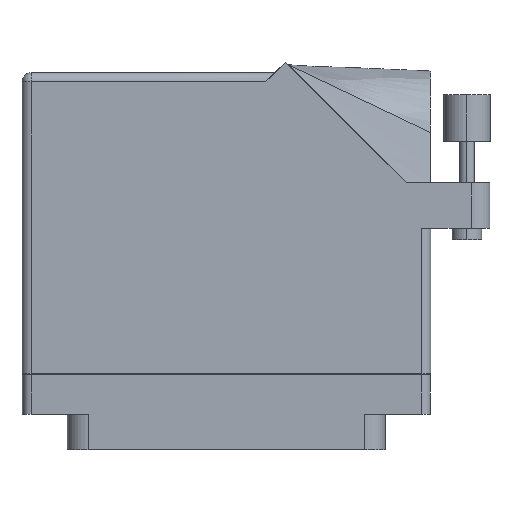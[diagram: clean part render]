
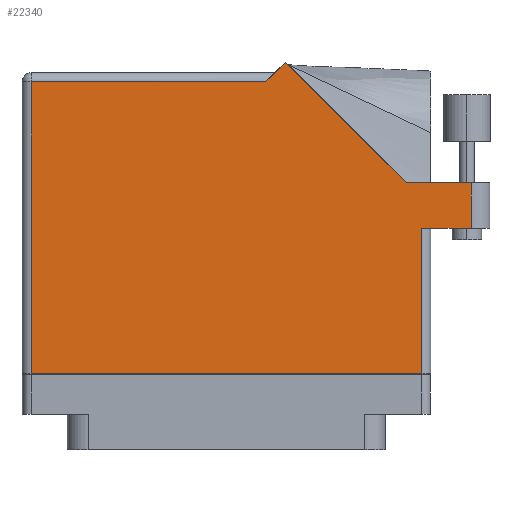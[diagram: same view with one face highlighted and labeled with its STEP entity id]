
A CAD part, front view. The second image highlights one B-rep face of the part: STEP entity #22340.
In plain terms, the highlighted face is planar.
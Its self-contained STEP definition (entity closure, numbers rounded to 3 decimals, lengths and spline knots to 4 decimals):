
#515 = CARTESIAN_POINT ( 'NONE',  ( 1.3155, 0.88, 0.765 ) ) ;
#1029 = CARTESIAN_POINT ( 'NONE',  ( 1.6525, 1.187, 0.765 ) ) ;
#1926 = DIRECTION ( 'NONE',  ( -1., 0., 0. ) ) ;
#1939 = VERTEX_POINT ( 'NONE', #44966 ) ;
#4307 = AXIS2_PLACEMENT_3D ( 'NONE', #61878, #61577, #21352 ) ;
#4882 = DIRECTION ( 'NONE',  ( -1., 0., 0. ) ) ;
#7314 = CARTESIAN_POINT ( 'NONE',  ( 1.6525, 0.88, 0.765 ) ) ;
#7640 = EDGE_CURVE ( 'NONE', #12763, #30041, #14751, .T. ) ;
#8707 = VERTEX_POINT ( 'NONE', #49635 ) ;
#8790 = VERTEX_POINT ( 'NONE', #7314 ) ;
#11628 = ORIENTED_EDGE ( 'NONE', *, *, #56207, .T. ) ;
#12763 = VERTEX_POINT ( 'NONE', #23673 ) ;
#14067 = PLANE ( 'NONE',  #4307 ) ;
#14723 = LINE ( 'NONE', #55177, #56525 ) ;
#14751 = LINE ( 'NONE', #14753, #34560 ) ;
#14753 = CARTESIAN_POINT ( 'NONE',  ( 1.7775, 1.187, 0.765 ) ) ;
#15245 = VERTEX_POINT ( 'NONE', #515 ) ;
#16291 = LINE ( 'NONE', #25675, #84075 ) ;
#16301 = EDGE_CURVE ( 'NONE', #30041, #19486, #49230, .T. ) ;
#17939 = VECTOR ( 'NONE', #72378, 39.3701 ) ;
#19486 = VERTEX_POINT ( 'NONE', #69228 ) ;
#20715 = LINE ( 'NONE', #1029, #49960 ) ;
#21352 = DIRECTION ( 'NONE',  ( -1., 0., 0. ) ) ;
#22222 = VECTOR ( 'NONE', #4882, 39.3701 ) ;
#22340 = ADVANCED_FACE ( 'NONE', ( #49860 ), #14067, .F. ) ;
#23673 = CARTESIAN_POINT ( 'NONE',  ( 1.6525, 1.187, 0.765 ) ) ;
#25675 = CARTESIAN_POINT ( 'NONE',  ( 1.3775, 0.88, 0.765 ) ) ;
#27542 = VECTOR ( 'NONE', #30844, 39.3701 ) ;
#30041 = VERTEX_POINT ( 'NONE', #47855 ) ;
#30844 = DIRECTION ( 'NONE',  ( 0., -1., 0. ) ) ;
#31288 = EDGE_CURVE ( 'NONE', #19486, #32441, #56195, .T. ) ;
#31578 = VECTOR ( 'NONE', #84535, 39.3701 ) ;
#32284 = ORIENTED_EDGE ( 'NONE', *, *, #31288, .T. ) ;
#32441 = VERTEX_POINT ( 'NONE', #76630 ) ;
#32853 = ORIENTED_EDGE ( 'NONE', *, *, #16301, .T. ) ;
#33890 = ORIENTED_EDGE ( 'NONE', *, *, #58969, .T. ) ;
#34560 = VECTOR ( 'NONE', #1926, 39.3701 ) ;
#37464 = VERTEX_POINT ( 'NONE', #38167 ) ;
#38167 = CARTESIAN_POINT ( 'NONE',  ( 1.3155, -0.1, 0.765 ) ) ;
#39055 = ORIENTED_EDGE ( 'NONE', *, *, #7640, .T. ) ;
#39727 = CARTESIAN_POINT ( 'NONE',  ( 1.2119, 1.187, 0.765 ) ) ;
#41301 = ORIENTED_EDGE ( 'NONE', *, *, #44675, .T. ) ;
#41952 = DIRECTION ( 'NONE',  ( -0.707, -0.707, 0. ) ) ;
#43632 = CARTESIAN_POINT ( 'NONE',  ( -1.3155, -0.1, 0.765 ) ) ;
#44675 = EDGE_CURVE ( 'NONE', #8790, #12763, #20715, .T. ) ;
#44916 = DIRECTION ( 'NONE',  ( 1., 0., 0. ) ) ;
#44966 = CARTESIAN_POINT ( 'NONE',  ( -1.3155, -0.1, 0.765 ) ) ;
#45659 = CARTESIAN_POINT ( 'NONE',  ( -1.3775, 1.868, 0.765 ) ) ;
#47855 = CARTESIAN_POINT ( 'NONE',  ( 1.2119, 1.187, 0.765 ) ) ;
#49230 = LINE ( 'NONE', #39727, #17939 ) ;
#49635 = CARTESIAN_POINT ( 'NONE',  ( -1.3155, 1.868, 0.765 ) ) ;
#49860 = FACE_OUTER_BOUND ( 'NONE', #55525, .T. ) ;
#49960 = VECTOR ( 'NONE', #81130, 39.3701 ) ;
#50570 = LINE ( 'NONE', #43632, #27542 ) ;
#50987 = VECTOR ( 'NONE', #41952, 39.3701 ) ;
#55177 = CARTESIAN_POINT ( 'NONE',  ( -1.3775, -0.1, 0.765 ) ) ;
#55525 = EDGE_LOOP ( 'NONE', ( #33890, #41301, #39055, #32853, #32284, #67363, #11628, #71183, #70630 ) ) ;
#56195 = LINE ( 'NONE', #67896, #50987 ) ;
#56207 = EDGE_CURVE ( 'NONE', #8707, #1939, #50570, .T. ) ;
#56525 = VECTOR ( 'NONE', #69153, 39.3701 ) ;
#57361 = EDGE_CURVE ( 'NONE', #37464, #15245, #80532, .T. ) ;
#57977 = EDGE_CURVE ( 'NONE', #1939, #37464, #14723, .T. ) ;
#58969 = EDGE_CURVE ( 'NONE', #15245, #8790, #16291, .T. ) ;
#61577 = DIRECTION ( 'NONE',  ( 0., 0., -1. ) ) ;
#61878 = CARTESIAN_POINT ( 'NONE',  ( -1.3775, 1.93, 0.765 ) ) ;
#67363 = ORIENTED_EDGE ( 'NONE', *, *, #84151, .T. ) ;
#67896 = CARTESIAN_POINT ( 'NONE',  ( 0.3275, 1.93, 0.765 ) ) ;
#69153 = DIRECTION ( 'NONE',  ( 1., 0., 0. ) ) ;
#69228 = CARTESIAN_POINT ( 'NONE',  ( 0.3982, 2.0007, 0.765 ) ) ;
#70630 = ORIENTED_EDGE ( 'NONE', *, *, #57361, .T. ) ;
#71183 = ORIENTED_EDGE ( 'NONE', *, *, #57977, .T. ) ;
#72378 = DIRECTION ( 'NONE',  ( -0.707, 0.707, 0. ) ) ;
#74317 = LINE ( 'NONE', #45659, #22222 ) ;
#76630 = CARTESIAN_POINT ( 'NONE',  ( 0.2655, 1.868, 0.765 ) ) ;
#78148 = CARTESIAN_POINT ( 'NONE',  ( 1.3155, 0.88, 0.765 ) ) ;
#80532 = LINE ( 'NONE', #78148, #31578 ) ;
#81130 = DIRECTION ( 'NONE',  ( 0., 1., 0. ) ) ;
#84075 = VECTOR ( 'NONE', #44916, 39.3701 ) ;
#84151 = EDGE_CURVE ( 'NONE', #32441, #8707, #74317, .T. ) ;
#84535 = DIRECTION ( 'NONE',  ( 0., 1., 0. ) ) ;
